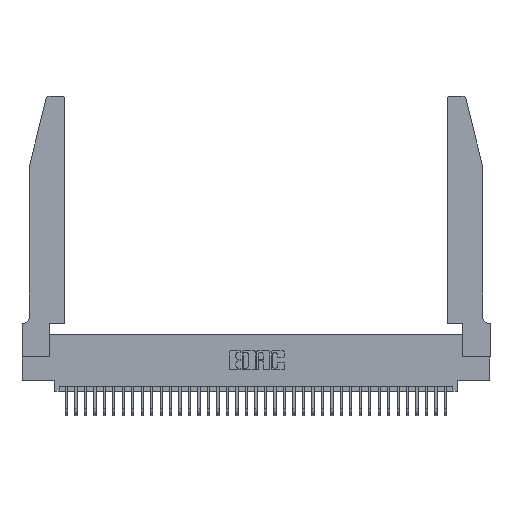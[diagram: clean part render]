
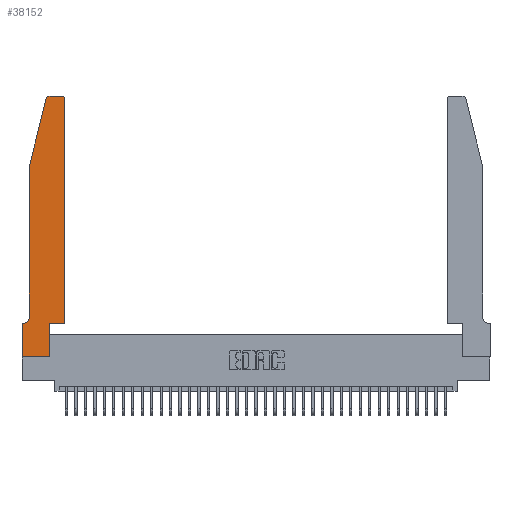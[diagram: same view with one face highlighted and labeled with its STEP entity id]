
A CAD part, top view. The second image highlights one B-rep face of the part: STEP entity #38152.
In plain terms, the highlighted planar face has unit normal (0, 0, 1).
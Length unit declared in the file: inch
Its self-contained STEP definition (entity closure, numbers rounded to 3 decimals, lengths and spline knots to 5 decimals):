
#978 = CARTESIAN_POINT ( 'NONE',  ( 0.4205, 2.75, 0.37 ) ) ;
#1607 = LINE ( 'NONE', #14081, #31616 ) ;
#1705 = CARTESIAN_POINT ( 'NONE',  ( 0.0755, 2., 0.37 ) ) ;
#1991 = AXIS2_PLACEMENT_3D ( 'NONE', #27742, #3519, #9414 ) ;
#2444 = EDGE_CURVE ( 'NONE', #26108, #27131, #29103, .T. ) ;
#2839 = ORIENTED_EDGE ( 'NONE', *, *, #10454, .T. ) ;
#3224 = EDGE_LOOP ( 'NONE', ( #30360, #12221, #35768, #23263, #31247, #33006, #32409, #23866, #2839, #14423, #25057, #29573 ) ) ;
#3307 = DIRECTION ( 'NONE',  ( 0., -1., 0. ) ) ;
#3324 = CARTESIAN_POINT ( 'NONE',  ( 0.0755, 0.42, 0.37 ) ) ;
#3344 = DIRECTION ( 'NONE',  ( 1., 0., 0. ) ) ;
#3451 = EDGE_CURVE ( 'NONE', #12801, #26108, #14476, .T. ) ;
#3519 = DIRECTION ( 'NONE',  ( 0., 0., -1. ) ) ;
#3549 = DIRECTION ( 'NONE',  ( 1., 0., 0. ) ) ;
#4436 = VERTEX_POINT ( 'NONE', #14083 ) ;
#4485 = VECTOR ( 'NONE', #25939, 39.37008 ) ;
#4931 = CARTESIAN_POINT ( 'NONE',  ( 0.4505, 2.72, 0.37 ) ) ;
#6215 = EDGE_CURVE ( 'NONE', #11241, #9334, #35337, .T. ) ;
#6762 = LINE ( 'NONE', #11485, #33515 ) ;
#8556 = EDGE_CURVE ( 'NONE', #4436, #34037, #15327, .T. ) ;
#9334 = VERTEX_POINT ( 'NONE', #13639 ) ;
#9338 = DIRECTION ( 'NONE',  ( 0., 1., 0. ) ) ;
#9414 = DIRECTION ( 'NONE',  ( -1., 0., 0. ) ) ;
#10454 = EDGE_CURVE ( 'NONE', #27131, #13672, #1607, .T. ) ;
#11241 = VERTEX_POINT ( 'NONE', #32007 ) ;
#11485 = CARTESIAN_POINT ( 'NONE',  ( 0.2605, 2.75, 0.37 ) ) ;
#11631 = CARTESIAN_POINT ( 'NONE',  ( 0., 0.35, 0.37 ) ) ;
#11781 = DIRECTION ( 'NONE',  ( 1., 0., 0. ) ) ;
#12221 = ORIENTED_EDGE ( 'NONE', *, *, #6215, .T. ) ;
#12801 = VERTEX_POINT ( 'NONE', #11631 ) ;
#13173 = DIRECTION ( 'NONE',  ( 0., 0., 1. ) ) ;
#13639 = CARTESIAN_POINT ( 'NONE',  ( 0.25487, 2.72718, 0.37 ) ) ;
#13672 = VERTEX_POINT ( 'NONE', #31482 ) ;
#14081 = CARTESIAN_POINT ( 'NONE',  ( 0.2865, 0.35, 0.37 ) ) ;
#14083 = CARTESIAN_POINT ( 'NONE',  ( 0.0755, 2., 0.37 ) ) ;
#14148 = DIRECTION ( 'NONE',  ( 1., 0., 0. ) ) ;
#14385 = CARTESIAN_POINT ( 'NONE',  ( 0.0055, 0.35, 0.37 ) ) ;
#14423 = ORIENTED_EDGE ( 'NONE', *, *, #18984, .T. ) ;
#14476 = LINE ( 'NONE', #29266, #27598 ) ;
#14895 = AXIS2_PLACEMENT_3D ( 'NONE', #15926, #13173, #27607 ) ;
#15327 = LINE ( 'NONE', #1705, #38356 ) ;
#15341 = CARTESIAN_POINT ( 'NONE',  ( 0.284, 2.72, 0.37 ) ) ;
#15926 = CARTESIAN_POINT ( 'NONE',  ( 0.4205, 2.72, 0.37 ) ) ;
#16375 = VERTEX_POINT ( 'NONE', #4931 ) ;
#16782 = PLANE ( 'NONE',  #29429 ) ;
#17135 = LINE ( 'NONE', #26704, #30263 ) ;
#17178 = CIRCLE ( 'NONE', #1991, 0.07 ) ;
#17517 = FACE_OUTER_BOUND ( 'NONE', #3224, .T. ) ;
#18613 = DIRECTION ( 'NONE',  ( 0., 0., 1. ) ) ;
#18984 = EDGE_CURVE ( 'NONE', #13672, #36612, #17135, .T. ) ;
#19634 = EDGE_CURVE ( 'NONE', #37212, #11241, #6762, .T. ) ;
#19817 = EDGE_CURVE ( 'NONE', #31360, #12801, #33485, .T. ) ;
#20204 = VECTOR ( 'NONE', #3344, 39.37008 ) ;
#20873 = LINE ( 'NONE', #24698, #38729 ) ;
#22867 = CARTESIAN_POINT ( 'NONE',  ( 0.4505, 0.35, 0.37 ) ) ;
#23263 = ORIENTED_EDGE ( 'NONE', *, *, #8556, .T. ) ;
#23866 = ORIENTED_EDGE ( 'NONE', *, *, #2444, .T. ) ;
#24698 = CARTESIAN_POINT ( 'NONE',  ( 0.4505, 0.35, 0.37 ) ) ;
#25057 = ORIENTED_EDGE ( 'NONE', *, *, #37173, .T. ) ;
#25939 = DIRECTION ( 'NONE',  ( -0.239, -0.971, 0. ) ) ;
#26108 = VERTEX_POINT ( 'NONE', #30712 ) ;
#26704 = CARTESIAN_POINT ( 'NONE',  ( 0.4505, 0.35, 0.37 ) ) ;
#27131 = VERTEX_POINT ( 'NONE', #32093 ) ;
#27474 = EDGE_CURVE ( 'NONE', #16375, #37212, #29326, .T. ) ;
#27598 = VECTOR ( 'NONE', #38491, 39.37008 ) ;
#27607 = DIRECTION ( 'NONE',  ( 1., 0., 0. ) ) ;
#27742 = CARTESIAN_POINT ( 'NONE',  ( 0.0055, 0.42, 0.37 ) ) ;
#28191 = AXIS2_PLACEMENT_3D ( 'NONE', #15341, #18613, #3549 ) ;
#29103 = LINE ( 'NONE', #36000, #20204 ) ;
#29266 = CARTESIAN_POINT ( 'NONE',  ( 0., 0., 0.37 ) ) ;
#29326 = CIRCLE ( 'NONE', #14895, 0.03 ) ;
#29429 = AXIS2_PLACEMENT_3D ( 'NONE', #34902, #37785, #14148 ) ;
#29573 = ORIENTED_EDGE ( 'NONE', *, *, #27474, .T. ) ;
#30216 = CARTESIAN_POINT ( 'NONE',  ( 0.0755, 0.35, 0.37 ) ) ;
#30263 = VECTOR ( 'NONE', #11781, 39.37008 ) ;
#30360 = ORIENTED_EDGE ( 'NONE', *, *, #19634, .T. ) ;
#30712 = CARTESIAN_POINT ( 'NONE',  ( 0., 0., 0.37 ) ) ;
#30859 = DIRECTION ( 'NONE',  ( 0., 1., 0. ) ) ;
#31247 = ORIENTED_EDGE ( 'NONE', *, *, #34756, .T. ) ;
#31360 = VERTEX_POINT ( 'NONE', #14385 ) ;
#31482 = CARTESIAN_POINT ( 'NONE',  ( 0.2865, 0.35, 0.37 ) ) ;
#31616 = VECTOR ( 'NONE', #9338, 39.37008 ) ;
#31900 = CARTESIAN_POINT ( 'NONE',  ( 0.0755, 2., 0.37 ) ) ;
#32007 = CARTESIAN_POINT ( 'NONE',  ( 0.284, 2.75, 0.37 ) ) ;
#32093 = CARTESIAN_POINT ( 'NONE',  ( 0.2865, 0., 0.37 ) ) ;
#32409 = ORIENTED_EDGE ( 'NONE', *, *, #3451, .T. ) ;
#33006 = ORIENTED_EDGE ( 'NONE', *, *, #19817, .T. ) ;
#33485 = LINE ( 'NONE', #30216, #37253 ) ;
#33515 = VECTOR ( 'NONE', #35623, 39.37008 ) ;
#33886 = DIRECTION ( 'NONE',  ( -1., 0., 0. ) ) ;
#34037 = VERTEX_POINT ( 'NONE', #3324 ) ;
#34756 = EDGE_CURVE ( 'NONE', #34037, #31360, #17178, .T. ) ;
#34902 = CARTESIAN_POINT ( 'NONE',  ( 0., 0.35, 0.37 ) ) ;
#35337 = CIRCLE ( 'NONE', #28191, 0.03 ) ;
#35623 = DIRECTION ( 'NONE',  ( -1., 0., 0. ) ) ;
#35768 = ORIENTED_EDGE ( 'NONE', *, *, #36633, .T. ) ;
#36000 = CARTESIAN_POINT ( 'NONE',  ( 0., 0., 0.37 ) ) ;
#36371 = LINE ( 'NONE', #31900, #4485 ) ;
#36612 = VERTEX_POINT ( 'NONE', #22867 ) ;
#36633 = EDGE_CURVE ( 'NONE', #9334, #4436, #36371, .T. ) ;
#37173 = EDGE_CURVE ( 'NONE', #36612, #16375, #20873, .T. ) ;
#37212 = VERTEX_POINT ( 'NONE', #978 ) ;
#37253 = VECTOR ( 'NONE', #33886, 39.37008 ) ;
#37785 = DIRECTION ( 'NONE',  ( 0., 0., 1. ) ) ;
#38152 = ADVANCED_FACE ( 'NONE', ( #17517 ), #16782, .T. ) ;
#38356 = VECTOR ( 'NONE', #3307, 39.37008 ) ;
#38491 = DIRECTION ( 'NONE',  ( 0., -1., 0. ) ) ;
#38729 = VECTOR ( 'NONE', #30859, 39.37008 ) ;
